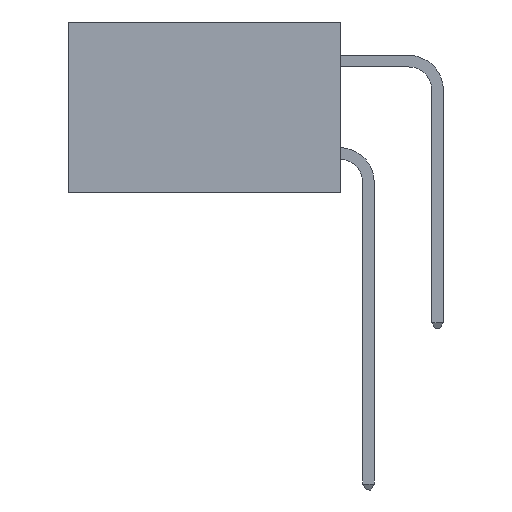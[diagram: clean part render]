
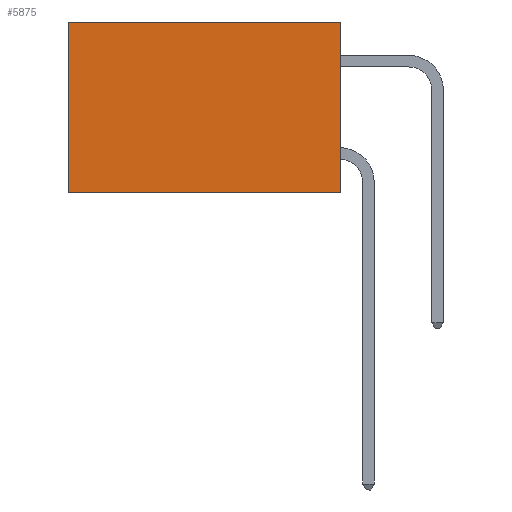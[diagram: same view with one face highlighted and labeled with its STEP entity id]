
A CAD part, left-side view. The second image highlights one B-rep face of the part: STEP entity #5875.
In plain terms, the highlighted planar face has unit normal (-1, 0, 0).
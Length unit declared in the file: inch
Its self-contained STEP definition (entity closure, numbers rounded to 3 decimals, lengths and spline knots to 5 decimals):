
#700 = VERTEX_POINT ( 'NONE', #7729 ) ;
#720 = ORIENTED_EDGE ( 'NONE', *, *, #9581, .F. ) ;
#1199 = EDGE_CURVE ( 'NONE', #9669, #700, #4202, .T. ) ;
#1782 = EDGE_CURVE ( 'NONE', #9669, #14946, #6361, .T. ) ;
#1918 = CARTESIAN_POINT ( 'NONE',  ( 0.277, 0., -0.37 ) ) ;
#2072 = CARTESIAN_POINT ( 'NONE',  ( 0.277, 0., 0. ) ) ;
#2601 = DIRECTION ( 'NONE',  ( 0., 0., -1. ) ) ;
#2742 = LINE ( 'NONE', #4451, #15507 ) ;
#2776 = CARTESIAN_POINT ( 'NONE',  ( 0.277, 0.59, -0.37 ) ) ;
#2857 = EDGE_LOOP ( 'NONE', ( #16221, #720, #5800, #7873 ) ) ;
#3013 = AXIS2_PLACEMENT_3D ( 'NONE', #3728, #13919, #6265 ) ;
#3138 = CARTESIAN_POINT ( 'NONE',  ( 0.277, 0., -0.37 ) ) ;
#3728 = CARTESIAN_POINT ( 'NONE',  ( 0.277, 0., -0.37 ) ) ;
#4202 = LINE ( 'NONE', #8740, #7592 ) ;
#4451 = CARTESIAN_POINT ( 'NONE',  ( 0.277, 0.59, -0.37 ) ) ;
#5800 = ORIENTED_EDGE ( 'NONE', *, *, #1782, .F. ) ;
#5867 = CARTESIAN_POINT ( 'NONE',  ( 0.277, 0., -0.37 ) ) ;
#5875 = ADVANCED_FACE ( 'NONE', ( #13840 ), #12623, .F. ) ;
#5955 = VECTOR ( 'NONE', #2601, 39.37008 ) ;
#6265 = DIRECTION ( 'NONE',  ( 0., 0., -1. ) ) ;
#6361 = LINE ( 'NONE', #1918, #5955 ) ;
#7333 = VECTOR ( 'NONE', #9566, 39.37008 ) ;
#7592 = VECTOR ( 'NONE', #10344, 39.37008 ) ;
#7729 = CARTESIAN_POINT ( 'NONE',  ( 0.277, 0.59, 0. ) ) ;
#7873 = ORIENTED_EDGE ( 'NONE', *, *, #1199, .T. ) ;
#8740 = CARTESIAN_POINT ( 'NONE',  ( 0.277, 0., 0. ) ) ;
#9566 = DIRECTION ( 'NONE',  ( 0., 1., 0. ) ) ;
#9581 = EDGE_CURVE ( 'NONE', #14946, #13184, #10742, .T. ) ;
#9669 = VERTEX_POINT ( 'NONE', #2072 ) ;
#10344 = DIRECTION ( 'NONE',  ( 0., 1., 0. ) ) ;
#10742 = LINE ( 'NONE', #3138, #7333 ) ;
#10794 = EDGE_CURVE ( 'NONE', #700, #13184, #2742, .T. ) ;
#12081 = DIRECTION ( 'NONE',  ( 0., 0., -1. ) ) ;
#12623 = PLANE ( 'NONE',  #3013 ) ;
#13184 = VERTEX_POINT ( 'NONE', #2776 ) ;
#13840 = FACE_OUTER_BOUND ( 'NONE', #2857, .T. ) ;
#13919 = DIRECTION ( 'NONE',  ( 1., 0., 0. ) ) ;
#14946 = VERTEX_POINT ( 'NONE', #5867 ) ;
#15507 = VECTOR ( 'NONE', #12081, 39.37008 ) ;
#16221 = ORIENTED_EDGE ( 'NONE', *, *, #10794, .T. ) ;
